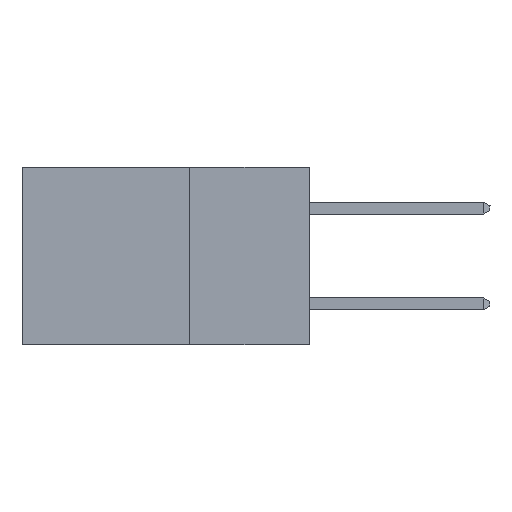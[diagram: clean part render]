
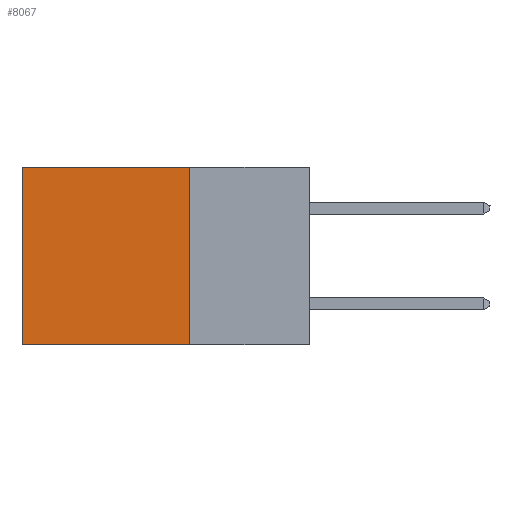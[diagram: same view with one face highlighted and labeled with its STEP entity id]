
A CAD part, left-side view. The second image highlights one B-rep face of the part: STEP entity #8067.
In plain terms, the highlighted planar face has unit normal (-1, 0, 0).
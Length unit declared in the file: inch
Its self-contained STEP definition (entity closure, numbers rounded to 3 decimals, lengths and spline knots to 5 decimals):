
#1910 = VECTOR ( 'NONE', #17105, 39.37008 ) ;
#2446 = LINE ( 'NONE', #20918, #11603 ) ;
#2755 = CARTESIAN_POINT ( 'NONE',  ( 0.2875, 0.25, 0. ) ) ;
#5476 = DIRECTION ( 'NONE',  ( 0., 1., 0. ) ) ;
#5649 = CARTESIAN_POINT ( 'NONE',  ( 0.2875, 0.25, 0. ) ) ;
#6117 = VERTEX_POINT ( 'NONE', #15810 ) ;
#6558 = ORIENTED_EDGE ( 'NONE', *, *, #27421, .T. ) ;
#6682 = ORIENTED_EDGE ( 'NONE', *, *, #28581, .T. ) ;
#7217 = FACE_OUTER_BOUND ( 'NONE', #7676, .T. ) ;
#7676 = EDGE_LOOP ( 'NONE', ( #6558, #10513, #24301, #6682 ) ) ;
#7777 = LINE ( 'NONE', #29156, #8637 ) ;
#8067 = ADVANCED_FACE ( 'NONE', ( #7217 ), #14093, .F. ) ;
#8637 = VECTOR ( 'NONE', #5476, 39.37008 ) ;
#10452 = CARTESIAN_POINT ( 'NONE',  ( 0.2875, 0.6, 0. ) ) ;
#10475 = DIRECTION ( 'NONE',  ( 0., 0., -1. ) ) ;
#10513 = ORIENTED_EDGE ( 'NONE', *, *, #24624, .F. ) ;
#11603 = VECTOR ( 'NONE', #16334, 39.37008 ) ;
#14093 = PLANE ( 'NONE',  #25079 ) ;
#15810 = CARTESIAN_POINT ( 'NONE',  ( 0.2875, 0.6, -0.37 ) ) ;
#16334 = DIRECTION ( 'NONE',  ( 0., 0., -1. ) ) ;
#16378 = DIRECTION ( 'NONE',  ( 1., 0., 0. ) ) ;
#16523 = DIRECTION ( 'NONE',  ( 0., 0., -1. ) ) ;
#17105 = DIRECTION ( 'NONE',  ( 0., 1., 0. ) ) ;
#18002 = VERTEX_POINT ( 'NONE', #10452 ) ;
#18264 = VECTOR ( 'NONE', #10475, 39.37008 ) ;
#19370 = EDGE_CURVE ( 'NONE', #24524, #26643, #20406, .T. ) ;
#20406 = LINE ( 'NONE', #24983, #18264 ) ;
#20918 = CARTESIAN_POINT ( 'NONE',  ( 0.2875, 0.6, 0. ) ) ;
#21414 = CARTESIAN_POINT ( 'NONE',  ( 0.2875, 0.25, 0. ) ) ;
#24301 = ORIENTED_EDGE ( 'NONE', *, *, #19370, .F. ) ;
#24524 = VERTEX_POINT ( 'NONE', #2755 ) ;
#24624 = EDGE_CURVE ( 'NONE', #26643, #6117, #7777, .T. ) ;
#24831 = CARTESIAN_POINT ( 'NONE',  ( 0.2875, 0.25, -0.37 ) ) ;
#24983 = CARTESIAN_POINT ( 'NONE',  ( 0.2875, 0.25, 0. ) ) ;
#25079 = AXIS2_PLACEMENT_3D ( 'NONE', #21414, #16378, #16523 ) ;
#26277 = LINE ( 'NONE', #5649, #1910 ) ;
#26643 = VERTEX_POINT ( 'NONE', #24831 ) ;
#27421 = EDGE_CURVE ( 'NONE', #18002, #6117, #2446, .T. ) ;
#28581 = EDGE_CURVE ( 'NONE', #24524, #18002, #26277, .T. ) ;
#29156 = CARTESIAN_POINT ( 'NONE',  ( 0.2875, 0.25, -0.37 ) ) ;
